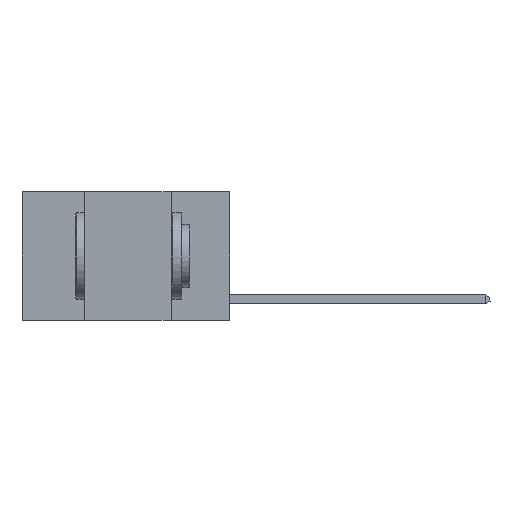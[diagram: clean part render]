
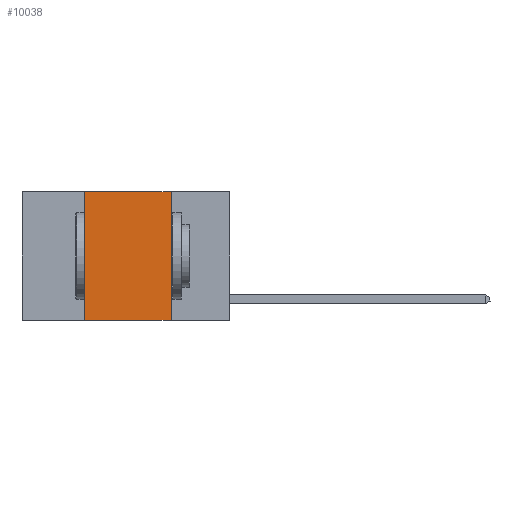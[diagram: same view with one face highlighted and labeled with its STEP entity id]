
A CAD part, left-side view. The second image highlights one B-rep face of the part: STEP entity #10038.
In plain terms, the highlighted planar face has unit normal (-1, 0, 0).
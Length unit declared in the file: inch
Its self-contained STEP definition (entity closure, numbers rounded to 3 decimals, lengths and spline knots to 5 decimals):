
#140 = DIRECTION ( 'NONE',  ( 0., 0., 1. ) ) ;
#788 = VERTEX_POINT ( 'NONE', #10677 ) ;
#1208 = EDGE_CURVE ( 'NONE', #8361, #788, #8418, .T. ) ;
#1511 = EDGE_CURVE ( 'NONE', #8805, #8361, #7150, .T. ) ;
#1717 = EDGE_CURVE ( 'NONE', #11670, #788, #9014, .T. ) ;
#2018 = VECTOR ( 'NONE', #11417, 39.37008 ) ;
#2198 = AXIS2_PLACEMENT_3D ( 'NONE', #5668, #3633, #6847 ) ;
#2276 = CARTESIAN_POINT ( 'NONE',  ( 0., 0.17, 0. ) ) ;
#2430 = PLANE ( 'NONE',  #2198 ) ;
#2669 = CARTESIAN_POINT ( 'NONE',  ( 0., 0.6, 0. ) ) ;
#3292 = VECTOR ( 'NONE', #4586, 39.37008 ) ;
#3621 = ORIENTED_EDGE ( 'NONE', *, *, #1208, .F. ) ;
#3633 = DIRECTION ( 'NONE',  ( 1., 0., 0. ) ) ;
#4437 = EDGE_LOOP ( 'NONE', ( #3621, #9959, #7303, #5623 ) ) ;
#4586 = DIRECTION ( 'NONE',  ( 0., -1., 0. ) ) ;
#5427 = EDGE_CURVE ( 'NONE', #11670, #8805, #6932, .T. ) ;
#5623 = ORIENTED_EDGE ( 'NONE', *, *, #1717, .T. ) ;
#5668 = CARTESIAN_POINT ( 'NONE',  ( 0., 0.6, 0. ) ) ;
#6288 = CARTESIAN_POINT ( 'NONE',  ( 0., 0.42, 0. ) ) ;
#6324 = VECTOR ( 'NONE', #6998, 39.37008 ) ;
#6847 = DIRECTION ( 'NONE',  ( 0., 0., -1. ) ) ;
#6932 = LINE ( 'NONE', #6288, #13022 ) ;
#6998 = DIRECTION ( 'NONE',  ( 0., -1., 0. ) ) ;
#7150 = LINE ( 'NONE', #2669, #3292 ) ;
#7303 = ORIENTED_EDGE ( 'NONE', *, *, #5427, .F. ) ;
#7692 = FACE_OUTER_BOUND ( 'NONE', #4437, .T. ) ;
#8361 = VERTEX_POINT ( 'NONE', #12313 ) ;
#8418 = LINE ( 'NONE', #2276, #2018 ) ;
#8805 = VERTEX_POINT ( 'NONE', #9138 ) ;
#8851 = CARTESIAN_POINT ( 'NONE',  ( 0., 0.6, -0.37 ) ) ;
#9014 = LINE ( 'NONE', #8851, #6324 ) ;
#9138 = CARTESIAN_POINT ( 'NONE',  ( 0., 0.42, 0. ) ) ;
#9959 = ORIENTED_EDGE ( 'NONE', *, *, #1511, .F. ) ;
#10038 = ADVANCED_FACE ( 'NONE', ( #7692 ), #2430, .F. ) ;
#10677 = CARTESIAN_POINT ( 'NONE',  ( 0., 0.17, -0.37 ) ) ;
#11417 = DIRECTION ( 'NONE',  ( 0., 0., -1. ) ) ;
#11670 = VERTEX_POINT ( 'NONE', #11782 ) ;
#11782 = CARTESIAN_POINT ( 'NONE',  ( 0., 0.42, -0.37 ) ) ;
#12313 = CARTESIAN_POINT ( 'NONE',  ( 0., 0.17, 0. ) ) ;
#13022 = VECTOR ( 'NONE', #140, 39.37008 ) ;
